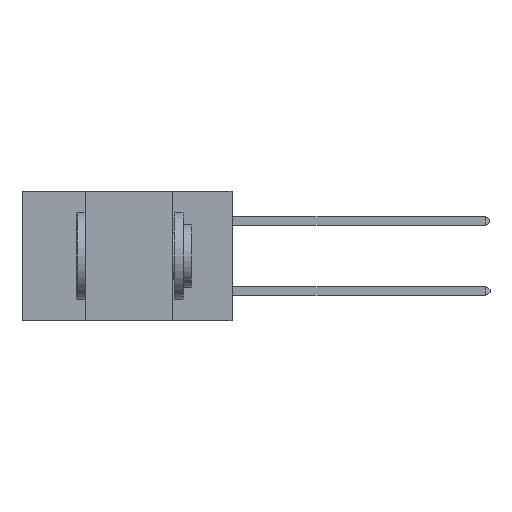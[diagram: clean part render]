
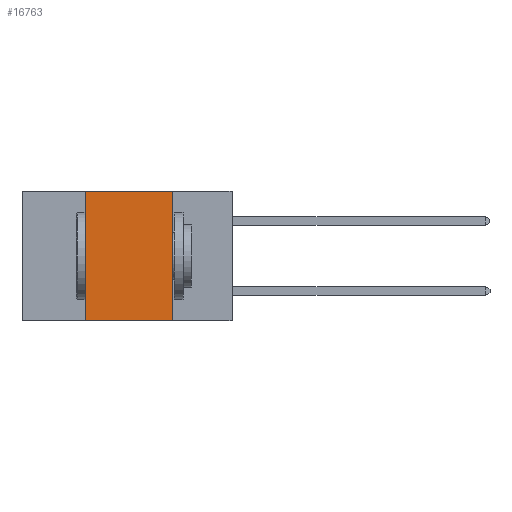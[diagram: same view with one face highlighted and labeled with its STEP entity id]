
A CAD part, left-side view. The second image highlights one B-rep face of the part: STEP entity #16763.
In plain terms, the highlighted planar face has unit normal (-1, 0, 0).
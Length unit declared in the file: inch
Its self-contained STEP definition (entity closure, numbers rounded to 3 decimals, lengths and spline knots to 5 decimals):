
#253 = DIRECTION ( 'NONE',  ( 1., 0., 0. ) ) ;
#420 = VERTEX_POINT ( 'NONE', #2882 ) ;
#1752 = LINE ( 'NONE', #14703, #15477 ) ;
#2882 = CARTESIAN_POINT ( 'NONE',  ( 0., 0.17, -0.37 ) ) ;
#3489 = VECTOR ( 'NONE', #22056, 39.37008 ) ;
#3511 = EDGE_CURVE ( 'NONE', #10578, #12798, #10291, .T. ) ;
#4027 = CARTESIAN_POINT ( 'NONE',  ( 0., 0.6, -0.37 ) ) ;
#4313 = ORIENTED_EDGE ( 'NONE', *, *, #7238, .F. ) ;
#4317 = EDGE_LOOP ( 'NONE', ( #7608, #4313, #13179, #22033 ) ) ;
#5210 = VECTOR ( 'NONE', #19586, 39.37008 ) ;
#5528 = LINE ( 'NONE', #4027, #3489 ) ;
#7238 = EDGE_CURVE ( 'NONE', #12798, #15294, #1752, .T. ) ;
#7608 = ORIENTED_EDGE ( 'NONE', *, *, #11328, .F. ) ;
#7730 = CARTESIAN_POINT ( 'NONE',  ( 0., 0.42, 0. ) ) ;
#8417 = EDGE_CURVE ( 'NONE', #10578, #420, #5528, .T. ) ;
#10291 = LINE ( 'NONE', #14038, #5210 ) ;
#10314 = AXIS2_PLACEMENT_3D ( 'NONE', #11378, #253, #15496 ) ;
#10399 = CARTESIAN_POINT ( 'NONE',  ( 0., 0.17, 0. ) ) ;
#10578 = VERTEX_POINT ( 'NONE', #23159 ) ;
#10789 = LINE ( 'NONE', #10399, #13170 ) ;
#11328 = EDGE_CURVE ( 'NONE', #15294, #420, #10789, .T. ) ;
#11378 = CARTESIAN_POINT ( 'NONE',  ( 0., 0.6, 0. ) ) ;
#12417 = CARTESIAN_POINT ( 'NONE',  ( 0., 0.17, 0. ) ) ;
#12798 = VERTEX_POINT ( 'NONE', #7730 ) ;
#13170 = VECTOR ( 'NONE', #14468, 39.37008 ) ;
#13179 = ORIENTED_EDGE ( 'NONE', *, *, #3511, .F. ) ;
#14038 = CARTESIAN_POINT ( 'NONE',  ( 0., 0.42, 0. ) ) ;
#14468 = DIRECTION ( 'NONE',  ( 0., 0., -1. ) ) ;
#14703 = CARTESIAN_POINT ( 'NONE',  ( 0., 0.6, 0. ) ) ;
#15294 = VERTEX_POINT ( 'NONE', #12417 ) ;
#15477 = VECTOR ( 'NONE', #20760, 39.37008 ) ;
#15496 = DIRECTION ( 'NONE',  ( 0., 0., -1. ) ) ;
#16763 = ADVANCED_FACE ( 'NONE', ( #23852 ), #21344, .F. ) ;
#19586 = DIRECTION ( 'NONE',  ( 0., 0., 1. ) ) ;
#20760 = DIRECTION ( 'NONE',  ( 0., -1., 0. ) ) ;
#21344 = PLANE ( 'NONE',  #10314 ) ;
#22033 = ORIENTED_EDGE ( 'NONE', *, *, #8417, .T. ) ;
#22056 = DIRECTION ( 'NONE',  ( 0., -1., 0. ) ) ;
#23159 = CARTESIAN_POINT ( 'NONE',  ( 0., 0.42, -0.37 ) ) ;
#23852 = FACE_OUTER_BOUND ( 'NONE', #4317, .T. ) ;
